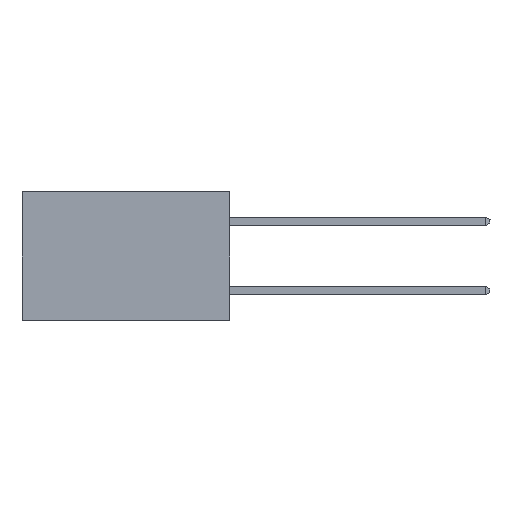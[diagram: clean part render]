
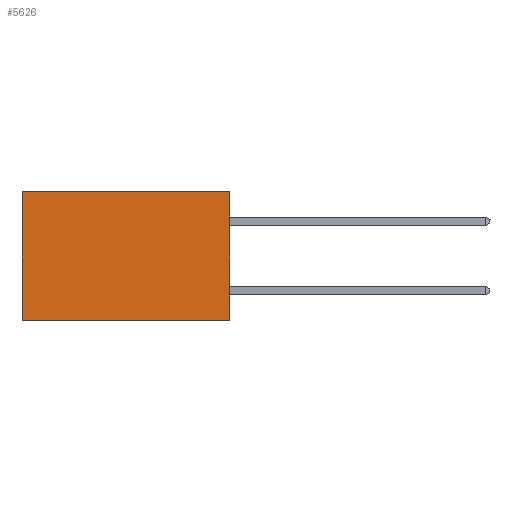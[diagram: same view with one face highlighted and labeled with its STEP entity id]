
A CAD part, left-side view. The second image highlights one B-rep face of the part: STEP entity #5626.
In plain terms, the highlighted planar face has unit normal (-1, 0, 0).
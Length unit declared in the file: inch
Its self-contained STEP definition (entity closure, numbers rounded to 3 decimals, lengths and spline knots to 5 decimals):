
#13 = EDGE_CURVE ( 'NONE', #4677, #8946, #4709, .T. ) ;
#242 = DIRECTION ( 'NONE',  ( 1., 0., 0. ) ) ;
#904 = VECTOR ( 'NONE', #8983, 39.37008 ) ;
#1004 = DIRECTION ( 'NONE',  ( 0., 0., -1. ) ) ;
#1214 = AXIS2_PLACEMENT_3D ( 'NONE', #8768, #242, #1228 ) ;
#1228 = DIRECTION ( 'NONE',  ( 0., 0., -1. ) ) ;
#1289 = EDGE_LOOP ( 'NONE', ( #4961, #3812, #7132, #7253 ) ) ;
#1473 = VECTOR ( 'NONE', #1004, 39.37008 ) ;
#1526 = LINE ( 'NONE', #5725, #3274 ) ;
#1599 = VECTOR ( 'NONE', #9680, 39.37008 ) ;
#2217 = CARTESIAN_POINT ( 'NONE',  ( 0.2615, 0., -0.37 ) ) ;
#2699 = CARTESIAN_POINT ( 'NONE',  ( 0.2615, 0.6, -0.37 ) ) ;
#2730 = EDGE_CURVE ( 'NONE', #6192, #4677, #1526, .T. ) ;
#3274 = VECTOR ( 'NONE', #4196, 39.37008 ) ;
#3771 = FACE_OUTER_BOUND ( 'NONE', #1289, .T. ) ;
#3812 = ORIENTED_EDGE ( 'NONE', *, *, #13, .F. ) ;
#3922 = LINE ( 'NONE', #6335, #1599 ) ;
#4168 = CARTESIAN_POINT ( 'NONE',  ( 0.2615, 0.6, 0. ) ) ;
#4196 = DIRECTION ( 'NONE',  ( 0., 0., -1. ) ) ;
#4590 = PLANE ( 'NONE',  #1214 ) ;
#4677 = VERTEX_POINT ( 'NONE', #10152 ) ;
#4709 = LINE ( 'NONE', #2217, #904 ) ;
#4961 = ORIENTED_EDGE ( 'NONE', *, *, #9182, .T. ) ;
#5626 = ADVANCED_FACE ( 'NONE', ( #3771 ), #4590, .F. ) ;
#5725 = CARTESIAN_POINT ( 'NONE',  ( 0.2615, 0., -0.37 ) ) ;
#5889 = VERTEX_POINT ( 'NONE', #4168 ) ;
#6192 = VERTEX_POINT ( 'NONE', #10508 ) ;
#6249 = EDGE_CURVE ( 'NONE', #6192, #5889, #3922, .T. ) ;
#6335 = CARTESIAN_POINT ( 'NONE',  ( 0.2615, 0., 0. ) ) ;
#7132 = ORIENTED_EDGE ( 'NONE', *, *, #2730, .F. ) ;
#7253 = ORIENTED_EDGE ( 'NONE', *, *, #6249, .T. ) ;
#8556 = LINE ( 'NONE', #2699, #1473 ) ;
#8768 = CARTESIAN_POINT ( 'NONE',  ( 0.2615, 0., -0.37 ) ) ;
#8832 = CARTESIAN_POINT ( 'NONE',  ( 0.2615, 0.6, -0.37 ) ) ;
#8946 = VERTEX_POINT ( 'NONE', #8832 ) ;
#8983 = DIRECTION ( 'NONE',  ( 0., 1., 0. ) ) ;
#9182 = EDGE_CURVE ( 'NONE', #5889, #8946, #8556, .T. ) ;
#9680 = DIRECTION ( 'NONE',  ( 0., 1., 0. ) ) ;
#10152 = CARTESIAN_POINT ( 'NONE',  ( 0.2615, 0., -0.37 ) ) ;
#10508 = CARTESIAN_POINT ( 'NONE',  ( 0.2615, 0., 0. ) ) ;
